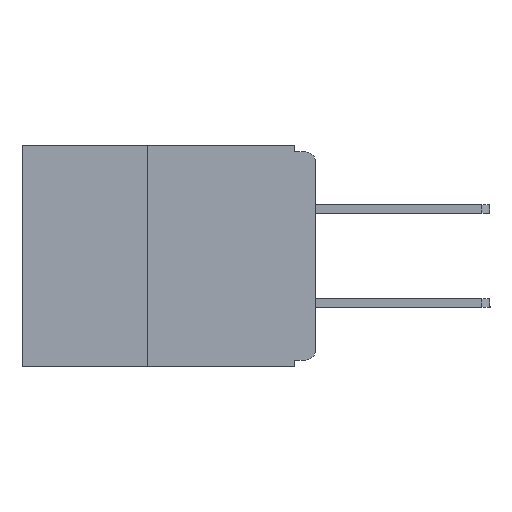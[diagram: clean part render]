
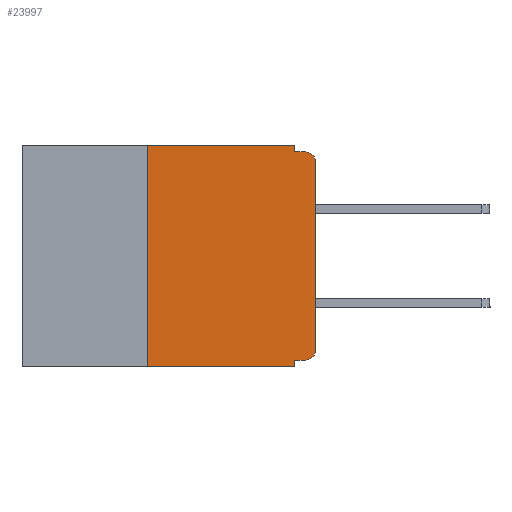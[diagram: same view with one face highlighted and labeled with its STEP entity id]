
A CAD part, left-side view. The second image highlights one B-rep face of the part: STEP entity #23997.
In plain terms, the highlighted planar face has unit normal (-1, 0, 0).
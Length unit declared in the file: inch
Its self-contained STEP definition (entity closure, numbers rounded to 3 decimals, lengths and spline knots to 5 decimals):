
#551 = VECTOR ( 'NONE', #14529, 39.37008 ) ;
#729 = LINE ( 'NONE', #25592, #12925 ) ;
#1064 = EDGE_CURVE ( 'NONE', #25985, #16749, #29700, .T. ) ;
#1387 = LINE ( 'NONE', #28155, #26517 ) ;
#1457 = ORIENTED_EDGE ( 'NONE', *, *, #11002, .T. ) ;
#1951 = VERTEX_POINT ( 'NONE', #17644 ) ;
#2638 = DIRECTION ( 'NONE',  ( 0., 0., 1. ) ) ;
#2978 = PLANE ( 'NONE',  #8445 ) ;
#3741 = CARTESIAN_POINT ( 'NONE',  ( 0., 0.031, -0.33 ) ) ;
#4101 = ORIENTED_EDGE ( 'NONE', *, *, #30360, .T. ) ;
#4165 = VERTEX_POINT ( 'NONE', #24795 ) ;
#5458 = DIRECTION ( 'NONE',  ( 1., 0., 0. ) ) ;
#5487 = VERTEX_POINT ( 'NONE', #25669 ) ;
#5994 = VERTEX_POINT ( 'NONE', #23295 ) ;
#6665 = DIRECTION ( 'NONE',  ( 0., 1., 0. ) ) ;
#7155 = EDGE_LOOP ( 'NONE', ( #4101, #25763, #27944, #14982, #14143, #9677, #1457, #31569, #16140, #17731 ) ) ;
#7290 = AXIS2_PLACEMENT_3D ( 'NONE', #9411, #26390, #11841 ) ;
#8445 = AXIS2_PLACEMENT_3D ( 'NONE', #17562, #5458, #22442 ) ;
#8651 = CARTESIAN_POINT ( 'NONE',  ( 0., 0.031, -0.33 ) ) ;
#9411 = CARTESIAN_POINT ( 'NONE',  ( 0., 0.015, -0.025 ) ) ;
#9677 = ORIENTED_EDGE ( 'NONE', *, *, #13608, .F. ) ;
#9866 = VECTOR ( 'NONE', #16671, 39.37008 ) ;
#9929 = FACE_OUTER_BOUND ( 'NONE', #7155, .T. ) ;
#9999 = EDGE_CURVE ( 'NONE', #5994, #13107, #10177, .T. ) ;
#10177 = LINE ( 'NONE', #8651, #10952 ) ;
#10952 = VECTOR ( 'NONE', #28068, 39.37008 ) ;
#11002 = EDGE_CURVE ( 'NONE', #1951, #13107, #19990, .T. ) ;
#11319 = VERTEX_POINT ( 'NONE', #13311 ) ;
#11841 = DIRECTION ( 'NONE',  ( 0., 0., -1. ) ) ;
#11864 = EDGE_CURVE ( 'NONE', #14670, #16749, #15772, .T. ) ;
#12079 = CARTESIAN_POINT ( 'NONE',  ( 0., 0.437, -0.33 ) ) ;
#12782 = DIRECTION ( 'NONE',  ( -1., 0., 0. ) ) ;
#12925 = VECTOR ( 'NONE', #13482, 39.37008 ) ;
#13107 = VERTEX_POINT ( 'NONE', #3741 ) ;
#13311 = CARTESIAN_POINT ( 'NONE',  ( 0., 0.015, -0.32 ) ) ;
#13316 = VECTOR ( 'NONE', #6665, 39.37008 ) ;
#13482 = DIRECTION ( 'NONE',  ( 0., 0., 1. ) ) ;
#13509 = DIRECTION ( 'NONE',  ( 0., -1., 0. ) ) ;
#13608 = EDGE_CURVE ( 'NONE', #1951, #22610, #24050, .T. ) ;
#13613 = DIRECTION ( 'NONE',  ( 0., 0., -1. ) ) ;
#14106 = LINE ( 'NONE', #23626, #13316 ) ;
#14143 = ORIENTED_EDGE ( 'NONE', *, *, #30926, .F. ) ;
#14529 = DIRECTION ( 'NONE',  ( 0., -1., 0. ) ) ;
#14670 = VERTEX_POINT ( 'NONE', #18758 ) ;
#14678 = EDGE_CURVE ( 'NONE', #11319, #5994, #14106, .T. ) ;
#14982 = ORIENTED_EDGE ( 'NONE', *, *, #19913, .F. ) ;
#15772 = LINE ( 'NONE', #28067, #22971 ) ;
#16140 = ORIENTED_EDGE ( 'NONE', *, *, #14678, .F. ) ;
#16543 = CARTESIAN_POINT ( 'NONE',  ( 0., 0., -0.025 ) ) ;
#16671 = DIRECTION ( 'NONE',  ( 0., -1., 0. ) ) ;
#16696 = CARTESIAN_POINT ( 'NONE',  ( 0., 0.25, 0. ) ) ;
#16749 = VERTEX_POINT ( 'NONE', #29894 ) ;
#17562 = CARTESIAN_POINT ( 'NONE',  ( 0., 0.437, 0. ) ) ;
#17644 = CARTESIAN_POINT ( 'NONE',  ( 0., 0.25, -0.33 ) ) ;
#17731 = ORIENTED_EDGE ( 'NONE', *, *, #29512, .T. ) ;
#18758 = CARTESIAN_POINT ( 'NONE',  ( 0., 0.031, -0.01 ) ) ;
#19913 = EDGE_CURVE ( 'NONE', #5487, #14670, #1387, .T. ) ;
#19990 = LINE ( 'NONE', #12079, #551 ) ;
#22442 = DIRECTION ( 'NONE',  ( 0., 0., -1. ) ) ;
#22517 = VECTOR ( 'NONE', #2638, 39.37008 ) ;
#22610 = VERTEX_POINT ( 'NONE', #16696 ) ;
#22893 = CIRCLE ( 'NONE', #27290, 0.015 ) ;
#22971 = VECTOR ( 'NONE', #13509, 39.37008 ) ;
#23295 = CARTESIAN_POINT ( 'NONE',  ( 0., 0.031, -0.32 ) ) ;
#23626 = CARTESIAN_POINT ( 'NONE',  ( 0., 0., -0.32 ) ) ;
#23877 = CARTESIAN_POINT ( 'NONE',  ( 0., 0.437, 0. ) ) ;
#23997 = ADVANCED_FACE ( 'NONE', ( #9929 ), #2978, .F. ) ;
#24050 = LINE ( 'NONE', #26892, #22517 ) ;
#24795 = CARTESIAN_POINT ( 'NONE',  ( 0., 0., -0.305 ) ) ;
#25592 = CARTESIAN_POINT ( 'NONE',  ( 0., 0., 0. ) ) ;
#25669 = CARTESIAN_POINT ( 'NONE',  ( 0., 0.031, 0. ) ) ;
#25763 = ORIENTED_EDGE ( 'NONE', *, *, #1064, .T. ) ;
#25985 = VERTEX_POINT ( 'NONE', #16543 ) ;
#26390 = DIRECTION ( 'NONE',  ( -1., 0., 0. ) ) ;
#26517 = VECTOR ( 'NONE', #13613, 39.37008 ) ;
#26892 = CARTESIAN_POINT ( 'NONE',  ( 0., 0.25, -0.33 ) ) ;
#27290 = AXIS2_PLACEMENT_3D ( 'NONE', #27345, #12782, #29794 ) ;
#27345 = CARTESIAN_POINT ( 'NONE',  ( 0., 0.015, -0.305 ) ) ;
#27944 = ORIENTED_EDGE ( 'NONE', *, *, #11864, .F. ) ;
#28068 = DIRECTION ( 'NONE',  ( 0., 0., -1. ) ) ;
#28067 = CARTESIAN_POINT ( 'NONE',  ( 0., 0., -0.01 ) ) ;
#28155 = CARTESIAN_POINT ( 'NONE',  ( 0., 0.031, 0. ) ) ;
#29259 = LINE ( 'NONE', #23877, #9866 ) ;
#29512 = EDGE_CURVE ( 'NONE', #11319, #4165, #22893, .T. ) ;
#29700 = CIRCLE ( 'NONE', #7290, 0.015 ) ;
#29794 = DIRECTION ( 'NONE',  ( 0., 0., -1. ) ) ;
#29894 = CARTESIAN_POINT ( 'NONE',  ( 0., 0.015, -0.01 ) ) ;
#30360 = EDGE_CURVE ( 'NONE', #4165, #25985, #729, .T. ) ;
#30926 = EDGE_CURVE ( 'NONE', #22610, #5487, #29259, .T. ) ;
#31569 = ORIENTED_EDGE ( 'NONE', *, *, #9999, .F. ) ;
